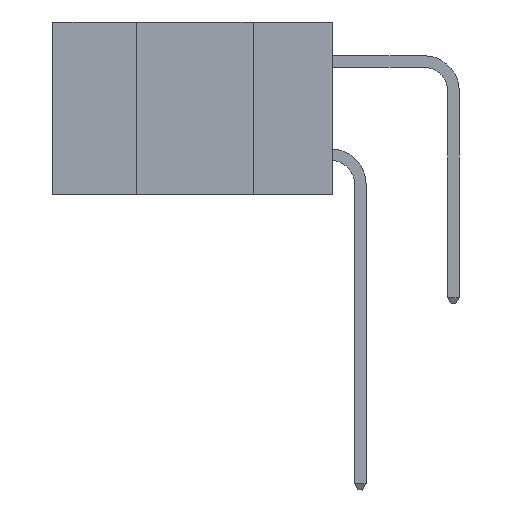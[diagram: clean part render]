
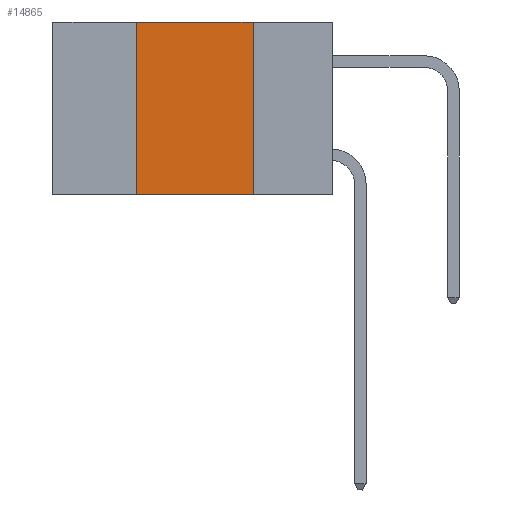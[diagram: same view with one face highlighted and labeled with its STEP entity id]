
A CAD part, left-side view. The second image highlights one B-rep face of the part: STEP entity #14865.
In plain terms, the highlighted planar face has unit normal (-1, 0, 0).
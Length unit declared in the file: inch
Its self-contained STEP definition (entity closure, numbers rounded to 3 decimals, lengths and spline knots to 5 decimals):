
#50 = EDGE_LOOP ( 'NONE', ( #335, #781, #14146, #4955 ) ) ;
#104 = DIRECTION ( 'NONE',  ( 0., -1., 0. ) ) ;
#335 = ORIENTED_EDGE ( 'NONE', *, *, #2436, .F. ) ;
#614 = CARTESIAN_POINT ( 'NONE',  ( 0., 0.6, 0. ) ) ;
#781 = ORIENTED_EDGE ( 'NONE', *, *, #4749, .F. ) ;
#1186 = VECTOR ( 'NONE', #16331, 39.37008 ) ;
#1198 = CARTESIAN_POINT ( 'NONE',  ( 0., 0.17, 0. ) ) ;
#1481 = LINE ( 'NONE', #17217, #17653 ) ;
#2087 = PLANE ( 'NONE',  #5480 ) ;
#2436 = EDGE_CURVE ( 'NONE', #7509, #18316, #17723, .T. ) ;
#2599 = VECTOR ( 'NONE', #104, 39.37008 ) ;
#3684 = DIRECTION ( 'NONE',  ( 1., 0., 0. ) ) ;
#4749 = EDGE_CURVE ( 'NONE', #5163, #7509, #9960, .T. ) ;
#4955 = ORIENTED_EDGE ( 'NONE', *, *, #10382, .T. ) ;
#5163 = VERTEX_POINT ( 'NONE', #13309 ) ;
#5480 = AXIS2_PLACEMENT_3D ( 'NONE', #614, #3684, #14397 ) ;
#7509 = VERTEX_POINT ( 'NONE', #1198 ) ;
#7848 = CARTESIAN_POINT ( 'NONE',  ( 0., 0.6, -0.37 ) ) ;
#8619 = CARTESIAN_POINT ( 'NONE',  ( 0., 0.17, 0. ) ) ;
#9830 = DIRECTION ( 'NONE',  ( 0., 0., 1. ) ) ;
#9960 = LINE ( 'NONE', #16442, #1186 ) ;
#10323 = CARTESIAN_POINT ( 'NONE',  ( 0., 0.17, -0.37 ) ) ;
#10382 = EDGE_CURVE ( 'NONE', #18659, #18316, #18706, .T. ) ;
#13309 = CARTESIAN_POINT ( 'NONE',  ( 0., 0.42, 0. ) ) ;
#14146 = ORIENTED_EDGE ( 'NONE', *, *, #14796, .F. ) ;
#14397 = DIRECTION ( 'NONE',  ( 0., 0., -1. ) ) ;
#14796 = EDGE_CURVE ( 'NONE', #18659, #5163, #1481, .T. ) ;
#14865 = ADVANCED_FACE ( 'NONE', ( #16250 ), #2087, .F. ) ;
#16250 = FACE_OUTER_BOUND ( 'NONE', #50, .T. ) ;
#16331 = DIRECTION ( 'NONE',  ( 0., -1., 0. ) ) ;
#16442 = CARTESIAN_POINT ( 'NONE',  ( 0., 0.6, 0. ) ) ;
#16933 = DIRECTION ( 'NONE',  ( 0., 0., -1. ) ) ;
#17217 = CARTESIAN_POINT ( 'NONE',  ( 0., 0.42, 0. ) ) ;
#17278 = VECTOR ( 'NONE', #16933, 39.37008 ) ;
#17653 = VECTOR ( 'NONE', #9830, 39.37008 ) ;
#17723 = LINE ( 'NONE', #8619, #17278 ) ;
#18316 = VERTEX_POINT ( 'NONE', #10323 ) ;
#18418 = CARTESIAN_POINT ( 'NONE',  ( 0., 0.42, -0.37 ) ) ;
#18659 = VERTEX_POINT ( 'NONE', #18418 ) ;
#18706 = LINE ( 'NONE', #7848, #2599 ) ;
